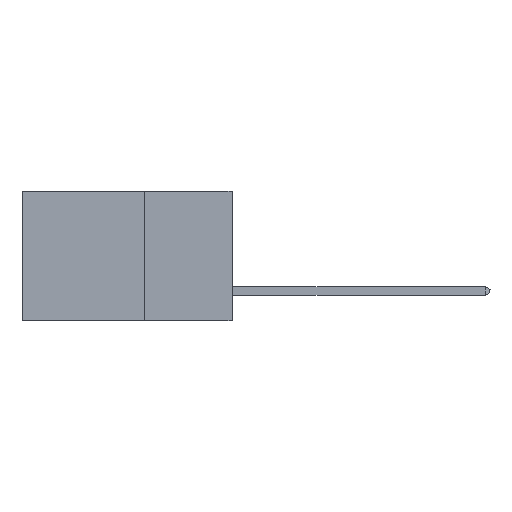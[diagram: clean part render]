
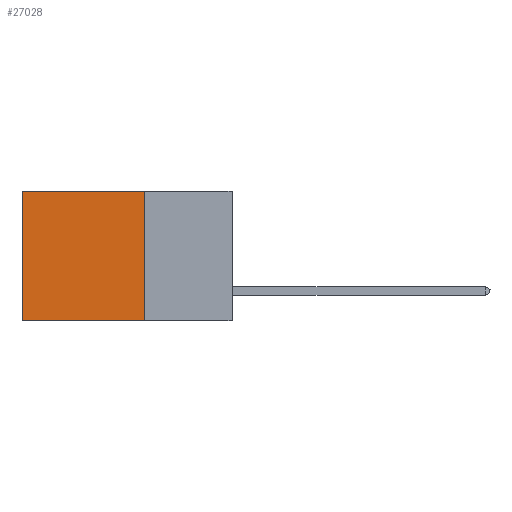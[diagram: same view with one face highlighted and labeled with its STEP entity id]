
A CAD part, left-side view. The second image highlights one B-rep face of the part: STEP entity #27028.
In plain terms, the highlighted planar face has unit normal (-1, 0, 0).
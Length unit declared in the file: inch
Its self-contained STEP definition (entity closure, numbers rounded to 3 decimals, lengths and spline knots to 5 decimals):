
#1790 = CARTESIAN_POINT ( 'NONE',  ( 0.2875, 0.6, 0. ) ) ;
#2387 = ORIENTED_EDGE ( 'NONE', *, *, #7226, .T. ) ;
#3949 = AXIS2_PLACEMENT_3D ( 'NONE', #35503, #21286, #6723 ) ;
#6238 = DIRECTION ( 'NONE',  ( 0., 0., -1. ) ) ;
#6723 = DIRECTION ( 'NONE',  ( 0., 0., -1. ) ) ;
#7226 = EDGE_CURVE ( 'NONE', #29385, #17541, #41018, .T. ) ;
#7508 = CARTESIAN_POINT ( 'NONE',  ( 0.2875, 0.25, 0. ) ) ;
#9488 = VERTEX_POINT ( 'NONE', #10088 ) ;
#10088 = CARTESIAN_POINT ( 'NONE',  ( 0.2875, 0.25, -0.37 ) ) ;
#11995 = ORIENTED_EDGE ( 'NONE', *, *, #42708, .T. ) ;
#12154 = ORIENTED_EDGE ( 'NONE', *, *, #36101, .F. ) ;
#16236 = CARTESIAN_POINT ( 'NONE',  ( 0.2875, 0.25, 0. ) ) ;
#16352 = EDGE_LOOP ( 'NONE', ( #2387, #18576, #12154, #11995 ) ) ;
#17541 = VERTEX_POINT ( 'NONE', #17621 ) ;
#17621 = CARTESIAN_POINT ( 'NONE',  ( 0.2875, 0.6, -0.37 ) ) ;
#18296 = DIRECTION ( 'NONE',  ( 0., 1., 0. ) ) ;
#18455 = CARTESIAN_POINT ( 'NONE',  ( 0.2875, 0.25, -0.37 ) ) ;
#18576 = ORIENTED_EDGE ( 'NONE', *, *, #32940, .F. ) ;
#20331 = DIRECTION ( 'NONE',  ( 0., 0., -1. ) ) ;
#21286 = DIRECTION ( 'NONE',  ( 1., 0., 0. ) ) ;
#26066 = LINE ( 'NONE', #18455, #45989 ) ;
#27028 = ADVANCED_FACE ( 'NONE', ( #45195 ), #46100, .F. ) ;
#28226 = CARTESIAN_POINT ( 'NONE',  ( 0.2875, 0.25, 0. ) ) ;
#29385 = VERTEX_POINT ( 'NONE', #1790 ) ;
#29697 = LINE ( 'NONE', #16236, #33189 ) ;
#30174 = VECTOR ( 'NONE', #20331, 39.37008 ) ;
#32940 = EDGE_CURVE ( 'NONE', #9488, #17541, #26066, .T. ) ;
#33189 = VECTOR ( 'NONE', #35653, 39.37008 ) ;
#33713 = VERTEX_POINT ( 'NONE', #7508 ) ;
#33853 = VECTOR ( 'NONE', #6238, 39.37008 ) ;
#35503 = CARTESIAN_POINT ( 'NONE',  ( 0.2875, 0.25, 0. ) ) ;
#35653 = DIRECTION ( 'NONE',  ( 0., 1., 0. ) ) ;
#36101 = EDGE_CURVE ( 'NONE', #33713, #9488, #38400, .T. ) ;
#38400 = LINE ( 'NONE', #28226, #33853 ) ;
#41018 = LINE ( 'NONE', #41815, #30174 ) ;
#41815 = CARTESIAN_POINT ( 'NONE',  ( 0.2875, 0.6, 0. ) ) ;
#42708 = EDGE_CURVE ( 'NONE', #33713, #29385, #29697, .T. ) ;
#45195 = FACE_OUTER_BOUND ( 'NONE', #16352, .T. ) ;
#45989 = VECTOR ( 'NONE', #18296, 39.37008 ) ;
#46100 = PLANE ( 'NONE',  #3949 ) ;
